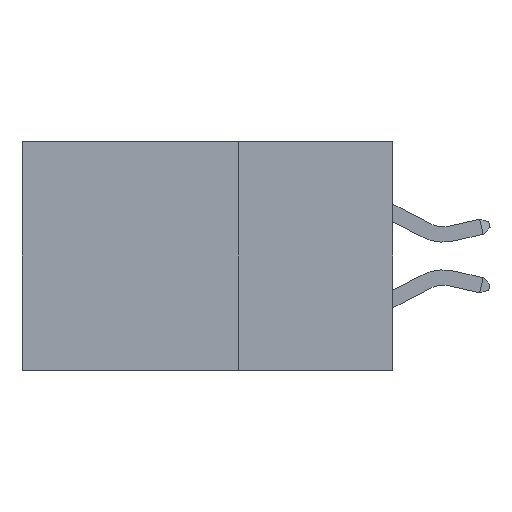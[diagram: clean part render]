
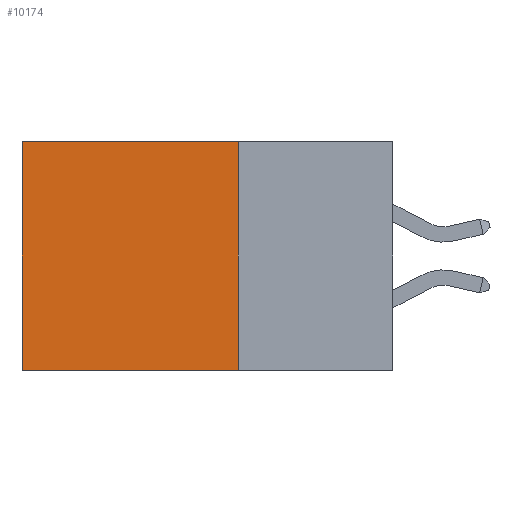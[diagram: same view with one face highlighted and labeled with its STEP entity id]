
A CAD part, left-side view. The second image highlights one B-rep face of the part: STEP entity #10174.
In plain terms, the highlighted planar face has unit normal (-1, 0, 0).
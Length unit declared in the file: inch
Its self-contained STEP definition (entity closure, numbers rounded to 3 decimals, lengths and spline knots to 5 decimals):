
#28 = ORIENTED_EDGE ( 'NONE', *, *, #2274, .T. ) ;
#854 = EDGE_LOOP ( 'NONE', ( #28, #24613, #7563, #8857 ) ) ;
#942 = EDGE_CURVE ( 'NONE', #14118, #18354, #12754, .T. ) ;
#1800 = CARTESIAN_POINT ( 'NONE',  ( 0.2875, 0.6, 0. ) ) ;
#2223 = CARTESIAN_POINT ( 'NONE',  ( 0.2875, 0.25, 0. ) ) ;
#2274 = EDGE_CURVE ( 'NONE', #22780, #18354, #12690, .T. ) ;
#2605 = VECTOR ( 'NONE', #22776, 39.37008 ) ;
#2852 = DIRECTION ( 'NONE',  ( 1., 0., 0. ) ) ;
#3905 = EDGE_CURVE ( 'NONE', #4348, #14118, #23545, .T. ) ;
#4348 = VERTEX_POINT ( 'NONE', #19640 ) ;
#4690 = DIRECTION ( 'NONE',  ( 0., 0., -1. ) ) ;
#5087 = CARTESIAN_POINT ( 'NONE',  ( 0.2875, 0.25, -0.37 ) ) ;
#6265 = VECTOR ( 'NONE', #10022, 39.37008 ) ;
#6880 = LINE ( 'NONE', #2223, #6265 ) ;
#7563 = ORIENTED_EDGE ( 'NONE', *, *, #3905, .F. ) ;
#7616 = CARTESIAN_POINT ( 'NONE',  ( 0.2875, 0.25, 0. ) ) ;
#8857 = ORIENTED_EDGE ( 'NONE', *, *, #12501, .T. ) ;
#10022 = DIRECTION ( 'NONE',  ( 0., 1., 0. ) ) ;
#10174 = ADVANCED_FACE ( 'NONE', ( #20199 ), #16109, .F. ) ;
#11380 = AXIS2_PLACEMENT_3D ( 'NONE', #19995, #2852, #16276 ) ;
#12501 = EDGE_CURVE ( 'NONE', #4348, #22780, #6880, .T. ) ;
#12690 = LINE ( 'NONE', #1800, #22130 ) ;
#12754 = LINE ( 'NONE', #15981, #22808 ) ;
#14118 = VERTEX_POINT ( 'NONE', #5087 ) ;
#15981 = CARTESIAN_POINT ( 'NONE',  ( 0.2875, 0.25, -0.37 ) ) ;
#16109 = PLANE ( 'NONE',  #11380 ) ;
#16151 = DIRECTION ( 'NONE',  ( 0., 1., 0. ) ) ;
#16276 = DIRECTION ( 'NONE',  ( 0., 0., -1. ) ) ;
#16906 = CARTESIAN_POINT ( 'NONE',  ( 0.2875, 0.6, -0.37 ) ) ;
#18354 = VERTEX_POINT ( 'NONE', #16906 ) ;
#19640 = CARTESIAN_POINT ( 'NONE',  ( 0.2875, 0.25, 0. ) ) ;
#19995 = CARTESIAN_POINT ( 'NONE',  ( 0.2875, 0.25, 0. ) ) ;
#20199 = FACE_OUTER_BOUND ( 'NONE', #854, .T. ) ;
#20567 = CARTESIAN_POINT ( 'NONE',  ( 0.2875, 0.6, 0. ) ) ;
#22130 = VECTOR ( 'NONE', #4690, 39.37008 ) ;
#22776 = DIRECTION ( 'NONE',  ( 0., 0., -1. ) ) ;
#22780 = VERTEX_POINT ( 'NONE', #20567 ) ;
#22808 = VECTOR ( 'NONE', #16151, 39.37008 ) ;
#23545 = LINE ( 'NONE', #7616, #2605 ) ;
#24613 = ORIENTED_EDGE ( 'NONE', *, *, #942, .F. ) ;
